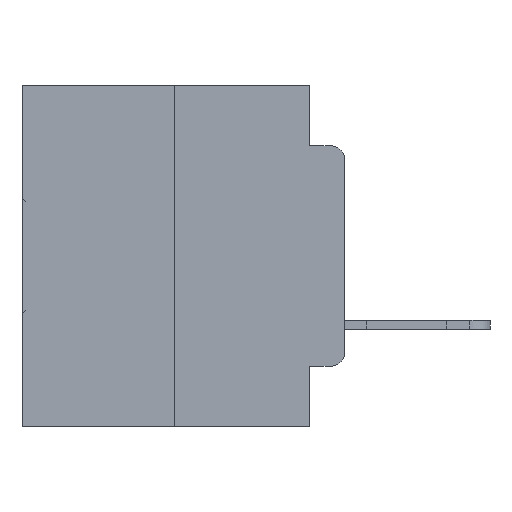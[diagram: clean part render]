
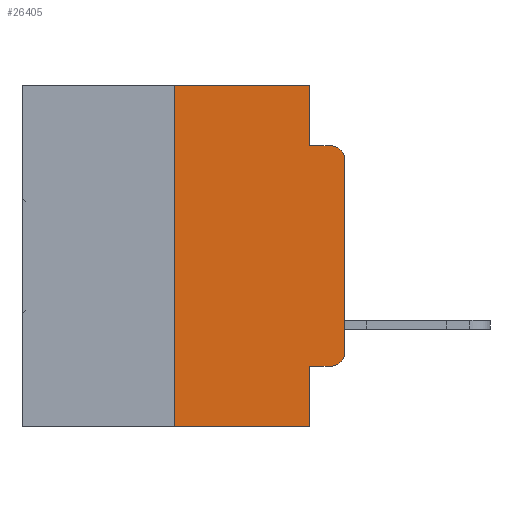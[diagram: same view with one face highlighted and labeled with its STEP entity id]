
A CAD part, left-side view. The second image highlights one B-rep face of the part: STEP entity #26405.
In plain terms, the highlighted planar face has unit normal (-1, 0, 0).
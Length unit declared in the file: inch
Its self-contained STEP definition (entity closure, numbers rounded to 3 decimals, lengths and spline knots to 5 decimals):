
#2 = CARTESIAN_POINT ( 'NONE',  ( 0., 0.473, -0.5 ) ) ;
#16 = EDGE_CURVE ( 'NONE', #2195, #12726, #9894, .T. ) ;
#327 = EDGE_CURVE ( 'NONE', #635, #16233, #26084, .T. ) ;
#488 = ORIENTED_EDGE ( 'NONE', *, *, #792, .T. ) ;
#635 = VERTEX_POINT ( 'NONE', #16567 ) ;
#696 = EDGE_CURVE ( 'NONE', #13745, #741, #28179, .T. ) ;
#741 = VERTEX_POINT ( 'NONE', #20780 ) ;
#792 = EDGE_CURVE ( 'NONE', #13745, #7425, #24713, .T. ) ;
#813 = FACE_OUTER_BOUND ( 'NONE', #5427, .T. ) ;
#1067 = EDGE_CURVE ( 'NONE', #7425, #25135, #25373, .T. ) ;
#1168 = LINE ( 'NONE', #2, #7307 ) ;
#1226 = CARTESIAN_POINT ( 'NONE',  ( 0., 0.02, -0.4115 ) ) ;
#1231 = CARTESIAN_POINT ( 'NONE',  ( 0., 0.051, 0. ) ) ;
#1472 = VECTOR ( 'NONE', #29905, 39.37008 ) ;
#1760 = DIRECTION ( 'NONE',  ( 0., 0., -1. ) ) ;
#1966 = VERTEX_POINT ( 'NONE', #30302 ) ;
#1993 = CARTESIAN_POINT ( 'NONE',  ( 0., 0.051, 0. ) ) ;
#2195 = VERTEX_POINT ( 'NONE', #1993 ) ;
#3186 = VECTOR ( 'NONE', #22273, 39.37008 ) ;
#3187 = VECTOR ( 'NONE', #1760, 39.37008 ) ;
#4200 = AXIS2_PLACEMENT_3D ( 'NONE', #6960, #27821, #14158 ) ;
#4950 = VERTEX_POINT ( 'NONE', #28893 ) ;
#5069 = CARTESIAN_POINT ( 'NONE',  ( 0., 0.02, -0.1085 ) ) ;
#5427 = EDGE_LOOP ( 'NONE', ( #14163, #8623, #21813, #27729, #17005, #29114, #18479, #30518, #488, #19964 ) ) ;
#6823 = CARTESIAN_POINT ( 'NONE',  ( 0., 0.051, -0.4115 ) ) ;
#6960 = CARTESIAN_POINT ( 'NONE',  ( 0., 0.473, 0. ) ) ;
#7307 = VECTOR ( 'NONE', #14937, 39.37008 ) ;
#7425 = VERTEX_POINT ( 'NONE', #1226 ) ;
#7584 = VECTOR ( 'NONE', #20132, 39.37008 ) ;
#7601 = DIRECTION ( 'NONE',  ( 0., 0., -1. ) ) ;
#7788 = EDGE_CURVE ( 'NONE', #16233, #2195, #11282, .T. ) ;
#8023 = CARTESIAN_POINT ( 'NONE',  ( 0., 0.473, 0. ) ) ;
#8623 = ORIENTED_EDGE ( 'NONE', *, *, #30727, .T. ) ;
#9894 = LINE ( 'NONE', #1231, #3187 ) ;
#11282 = LINE ( 'NONE', #8023, #28803 ) ;
#12422 = VECTOR ( 'NONE', #20439, 39.37008 ) ;
#12726 = VERTEX_POINT ( 'NONE', #22318 ) ;
#13372 = EDGE_CURVE ( 'NONE', #635, #741, #1168, .T. ) ;
#13739 = CARTESIAN_POINT ( 'NONE',  ( 0., 0.051, 0. ) ) ;
#13745 = VERTEX_POINT ( 'NONE', #6823 ) ;
#13807 = DIRECTION ( 'NONE',  ( 0., 0., -1. ) ) ;
#14158 = DIRECTION ( 'NONE',  ( 0., 0., -1. ) ) ;
#14163 = ORIENTED_EDGE ( 'NONE', *, *, #14931, .T. ) ;
#14931 = EDGE_CURVE ( 'NONE', #25135, #4950, #26113, .T. ) ;
#14937 = DIRECTION ( 'NONE',  ( 0., -1., 0. ) ) ;
#15198 = AXIS2_PLACEMENT_3D ( 'NONE', #5069, #21678, #7601 ) ;
#15494 = DIRECTION ( 'NONE',  ( 0., 0., -1. ) ) ;
#16233 = VERTEX_POINT ( 'NONE', #26942 ) ;
#16330 = PLANE ( 'NONE',  #4200 ) ;
#16567 = CARTESIAN_POINT ( 'NONE',  ( 0., 0.25, -0.5 ) ) ;
#17005 = ORIENTED_EDGE ( 'NONE', *, *, #7788, .F. ) ;
#18479 = ORIENTED_EDGE ( 'NONE', *, *, #13372, .T. ) ;
#19897 = CARTESIAN_POINT ( 'NONE',  ( 0., 0.051, -0.0885 ) ) ;
#19964 = ORIENTED_EDGE ( 'NONE', *, *, #1067, .T. ) ;
#19970 = CARTESIAN_POINT ( 'NONE',  ( 0., 0.051, -0.4115 ) ) ;
#20132 = DIRECTION ( 'NONE',  ( 0., 0., 1. ) ) ;
#20439 = DIRECTION ( 'NONE',  ( 0., -1., 0. ) ) ;
#20760 = CIRCLE ( 'NONE', #15198, 0.02 ) ;
#20780 = CARTESIAN_POINT ( 'NONE',  ( 0., 0.051, -0.5 ) ) ;
#21502 = CARTESIAN_POINT ( 'NONE',  ( 0., 0.25, 0. ) ) ;
#21678 = DIRECTION ( 'NONE',  ( -1., 0., 0. ) ) ;
#21813 = ORIENTED_EDGE ( 'NONE', *, *, #29227, .F. ) ;
#22273 = DIRECTION ( 'NONE',  ( 0., -1., 0. ) ) ;
#22292 = LINE ( 'NONE', #19897, #3186 ) ;
#22318 = CARTESIAN_POINT ( 'NONE',  ( 0., 0.051, -0.0885 ) ) ;
#22508 = CARTESIAN_POINT ( 'NONE',  ( 0., 0., 0. ) ) ;
#23978 = AXIS2_PLACEMENT_3D ( 'NONE', #30663, #26148, #15494 ) ;
#24306 = DIRECTION ( 'NONE',  ( 0., -1., 0. ) ) ;
#24713 = LINE ( 'NONE', #19970, #12422 ) ;
#25135 = VERTEX_POINT ( 'NONE', #27903 ) ;
#25373 = CIRCLE ( 'NONE', #23978, 0.02 ) ;
#26084 = LINE ( 'NONE', #21502, #1472 ) ;
#26113 = LINE ( 'NONE', #22508, #7584 ) ;
#26148 = DIRECTION ( 'NONE',  ( -1., 0., 0. ) ) ;
#26405 = ADVANCED_FACE ( 'NONE', ( #813 ), #16330, .F. ) ;
#26942 = CARTESIAN_POINT ( 'NONE',  ( 0., 0.25, 0. ) ) ;
#27495 = VECTOR ( 'NONE', #13807, 39.37008 ) ;
#27729 = ORIENTED_EDGE ( 'NONE', *, *, #16, .F. ) ;
#27821 = DIRECTION ( 'NONE',  ( 1., 0., 0. ) ) ;
#27903 = CARTESIAN_POINT ( 'NONE',  ( 0., 0., -0.3915 ) ) ;
#28179 = LINE ( 'NONE', #13739, #27495 ) ;
#28803 = VECTOR ( 'NONE', #24306, 39.37008 ) ;
#28893 = CARTESIAN_POINT ( 'NONE',  ( 0., 0., -0.1085 ) ) ;
#29114 = ORIENTED_EDGE ( 'NONE', *, *, #327, .F. ) ;
#29227 = EDGE_CURVE ( 'NONE', #12726, #1966, #22292, .T. ) ;
#29905 = DIRECTION ( 'NONE',  ( 0., 0., 1. ) ) ;
#30302 = CARTESIAN_POINT ( 'NONE',  ( 0., 0.02, -0.0885 ) ) ;
#30518 = ORIENTED_EDGE ( 'NONE', *, *, #696, .F. ) ;
#30663 = CARTESIAN_POINT ( 'NONE',  ( 0., 0.02, -0.3915 ) ) ;
#30727 = EDGE_CURVE ( 'NONE', #4950, #1966, #20760, .T. ) ;
